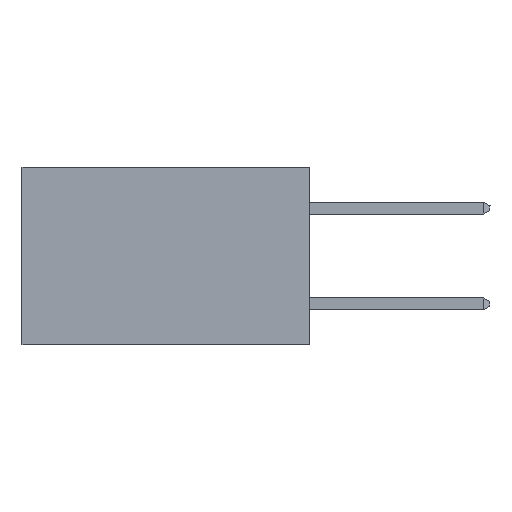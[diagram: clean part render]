
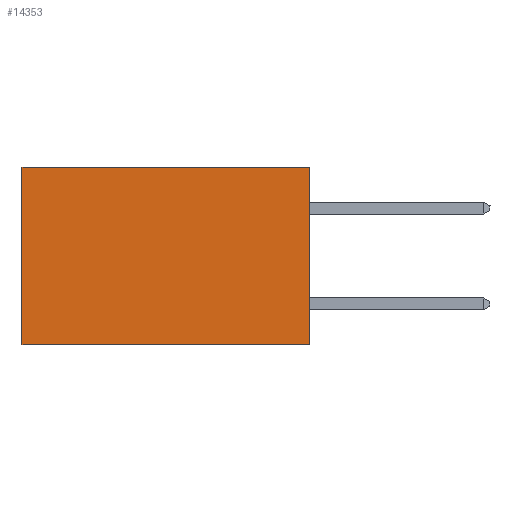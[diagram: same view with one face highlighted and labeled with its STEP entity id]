
A CAD part, left-side view. The second image highlights one B-rep face of the part: STEP entity #14353.
In plain terms, the highlighted planar face has unit normal (-1, 0, 0).
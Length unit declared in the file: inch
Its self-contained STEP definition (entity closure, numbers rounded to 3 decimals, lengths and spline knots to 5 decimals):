
#28 = CARTESIAN_POINT ( 'NONE',  ( 0.2875, 0., 0. ) ) ;
#438 = EDGE_CURVE ( 'NONE', #10962, #9479, #3679, .T. ) ;
#1606 = VECTOR ( 'NONE', #16804, 39.37008 ) ;
#1639 = PLANE ( 'NONE',  #4154 ) ;
#2847 = EDGE_CURVE ( 'NONE', #10433, #13870, #5691, .T. ) ;
#3104 = ORIENTED_EDGE ( 'NONE', *, *, #11374, .T. ) ;
#3370 = CARTESIAN_POINT ( 'NONE',  ( 0.2875, 0., -0.37 ) ) ;
#3659 = ORIENTED_EDGE ( 'NONE', *, *, #4257, .F. ) ;
#3679 = LINE ( 'NONE', #14314, #18614 ) ;
#4154 = AXIS2_PLACEMENT_3D ( 'NONE', #28, #4742, #14949 ) ;
#4257 = EDGE_CURVE ( 'NONE', #13870, #9479, #9344, .T. ) ;
#4742 = DIRECTION ( 'NONE',  ( 1., 0., 0. ) ) ;
#4940 = ORIENTED_EDGE ( 'NONE', *, *, #438, .T. ) ;
#5079 = DIRECTION ( 'NONE',  ( 0., 0., -1. ) ) ;
#5691 = LINE ( 'NONE', #18191, #1606 ) ;
#5696 = EDGE_LOOP ( 'NONE', ( #4940, #3659, #10131, #3104 ) ) ;
#6369 = CARTESIAN_POINT ( 'NONE',  ( 0.2875, 0., 0. ) ) ;
#7072 = VECTOR ( 'NONE', #7867, 39.37008 ) ;
#7090 = DIRECTION ( 'NONE',  ( 0., 1., 0. ) ) ;
#7423 = FACE_OUTER_BOUND ( 'NONE', #5696, .T. ) ;
#7867 = DIRECTION ( 'NONE',  ( 0., 1., 0. ) ) ;
#9344 = LINE ( 'NONE', #16874, #16493 ) ;
#9479 = VERTEX_POINT ( 'NONE', #13669 ) ;
#10131 = ORIENTED_EDGE ( 'NONE', *, *, #2847, .F. ) ;
#10221 = CARTESIAN_POINT ( 'NONE',  ( 0.2875, 0., 0. ) ) ;
#10433 = VERTEX_POINT ( 'NONE', #10221 ) ;
#10962 = VERTEX_POINT ( 'NONE', #12730 ) ;
#11374 = EDGE_CURVE ( 'NONE', #10433, #10962, #14796, .T. ) ;
#12730 = CARTESIAN_POINT ( 'NONE',  ( 0.2875, 0.6, 0. ) ) ;
#13669 = CARTESIAN_POINT ( 'NONE',  ( 0.2875, 0.6, -0.37 ) ) ;
#13870 = VERTEX_POINT ( 'NONE', #3370 ) ;
#14314 = CARTESIAN_POINT ( 'NONE',  ( 0.2875, 0.6, 0. ) ) ;
#14353 = ADVANCED_FACE ( 'NONE', ( #7423 ), #1639, .F. ) ;
#14796 = LINE ( 'NONE', #6369, #7072 ) ;
#14949 = DIRECTION ( 'NONE',  ( 0., 0., -1. ) ) ;
#16493 = VECTOR ( 'NONE', #7090, 39.37008 ) ;
#16804 = DIRECTION ( 'NONE',  ( 0., 0., -1. ) ) ;
#16874 = CARTESIAN_POINT ( 'NONE',  ( 0.2875, 0., -0.37 ) ) ;
#18191 = CARTESIAN_POINT ( 'NONE',  ( 0.2875, 0., 0. ) ) ;
#18614 = VECTOR ( 'NONE', #5079, 39.37008 ) ;
